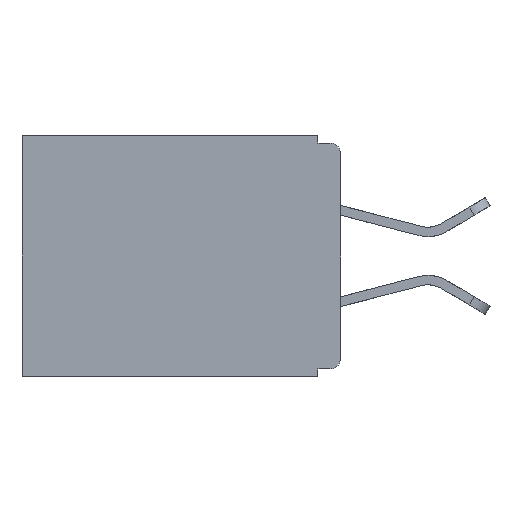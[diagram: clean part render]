
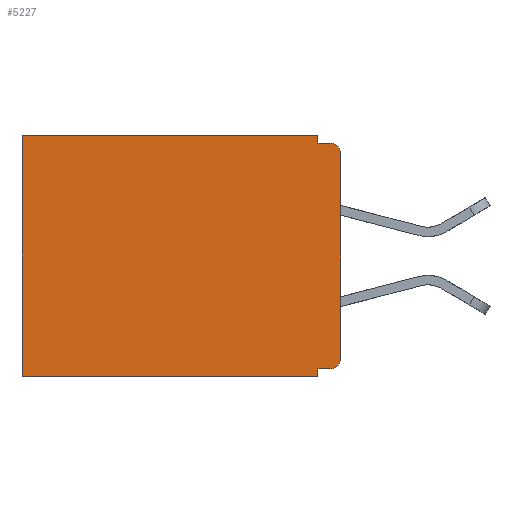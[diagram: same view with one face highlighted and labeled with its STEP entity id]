
A CAD part, left-side view. The second image highlights one B-rep face of the part: STEP entity #5227.
In plain terms, the highlighted planar face has unit normal (-1, 0, 0).
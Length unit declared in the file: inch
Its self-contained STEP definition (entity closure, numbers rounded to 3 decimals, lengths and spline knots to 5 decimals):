
#368 = VERTEX_POINT ( 'NONE', #8311 ) ;
#530 = VERTEX_POINT ( 'NONE', #10946 ) ;
#585 = AXIS2_PLACEMENT_3D ( 'NONE', #1080, #3379, #8536 ) ;
#915 = VERTEX_POINT ( 'NONE', #3968 ) ;
#994 = CARTESIAN_POINT ( 'NONE',  ( 0.3, 0., -0.33 ) ) ;
#1080 = CARTESIAN_POINT ( 'NONE',  ( 0.3, 0.015, -0.305 ) ) ;
#1088 = EDGE_CURVE ( 'NONE', #9975, #915, #9364, .T. ) ;
#1095 = ORIENTED_EDGE ( 'NONE', *, *, #3315, .F. ) ;
#1232 = LINE ( 'NONE', #8206, #9910 ) ;
#1527 = ORIENTED_EDGE ( 'NONE', *, *, #5737, .F. ) ;
#1800 = ORIENTED_EDGE ( 'NONE', *, *, #7945, .T. ) ;
#2013 = EDGE_CURVE ( 'NONE', #6006, #915, #11269, .T. ) ;
#2348 = CARTESIAN_POINT ( 'NONE',  ( 0.3, 0.437, -0.33 ) ) ;
#2437 = EDGE_LOOP ( 'NONE', ( #8509, #5768, #5359, #13763, #1800, #11108, #1527, #12391, #1095, #11787 ) ) ;
#2526 = LINE ( 'NONE', #6391, #11180 ) ;
#2609 = VECTOR ( 'NONE', #4242, 39.37008 ) ;
#2669 = CARTESIAN_POINT ( 'NONE',  ( 0.3, 0.031, -0.33 ) ) ;
#3148 = EDGE_CURVE ( 'NONE', #6006, #14381, #8460, .T. ) ;
#3163 = VECTOR ( 'NONE', #3804, 39.37008 ) ;
#3315 = EDGE_CURVE ( 'NONE', #9975, #7925, #3990, .T. ) ;
#3379 = DIRECTION ( 'NONE',  ( -1., 0., 0. ) ) ;
#3409 = VECTOR ( 'NONE', #7066, 39.37008 ) ;
#3683 = CARTESIAN_POINT ( 'NONE',  ( 0.3, 0., -0.32 ) ) ;
#3804 = DIRECTION ( 'NONE',  ( 0., 0., -1. ) ) ;
#3898 = DIRECTION ( 'NONE',  ( 0., 1., 0. ) ) ;
#3952 = CARTESIAN_POINT ( 'NONE',  ( 0.3, 0.031, -0.33 ) ) ;
#3968 = CARTESIAN_POINT ( 'NONE',  ( 0.3, 0., -0.305 ) ) ;
#3990 = LINE ( 'NONE', #3683, #6693 ) ;
#4228 = CARTESIAN_POINT ( 'NONE',  ( 0.3, 0., -0.33 ) ) ;
#4242 = DIRECTION ( 'NONE',  ( 0., 0., -1. ) ) ;
#4567 = VERTEX_POINT ( 'NONE', #3952 ) ;
#5057 = CARTESIAN_POINT ( 'NONE',  ( 0.3, 0.015, -0.01 ) ) ;
#5060 = CARTESIAN_POINT ( 'NONE',  ( 0.3, 0.031, -0.32 ) ) ;
#5227 = ADVANCED_FACE ( 'NONE', ( #8764 ), #5951, .F. ) ;
#5359 = ORIENTED_EDGE ( 'NONE', *, *, #6776, .F. ) ;
#5534 = EDGE_CURVE ( 'NONE', #6326, #8712, #2526, .T. ) ;
#5685 = CARTESIAN_POINT ( 'NONE',  ( 0.3, 0.437, 0. ) ) ;
#5737 = EDGE_CURVE ( 'NONE', #4567, #8712, #11700, .T. ) ;
#5768 = ORIENTED_EDGE ( 'NONE', *, *, #3148, .T. ) ;
#5951 = PLANE ( 'NONE',  #8265 ) ;
#6006 = VERTEX_POINT ( 'NONE', #10022 ) ;
#6097 = VECTOR ( 'NONE', #13013, 39.37008 ) ;
#6257 = LINE ( 'NONE', #2669, #3163 ) ;
#6326 = VERTEX_POINT ( 'NONE', #5685 ) ;
#6391 = CARTESIAN_POINT ( 'NONE',  ( 0.3, 0.437, -0.33 ) ) ;
#6445 = AXIS2_PLACEMENT_3D ( 'NONE', #10633, #7828, #7995 ) ;
#6693 = VECTOR ( 'NONE', #10478, 39.37008 ) ;
#6776 = EDGE_CURVE ( 'NONE', #530, #14381, #7347, .T. ) ;
#7066 = DIRECTION ( 'NONE',  ( 0., 1., 0. ) ) ;
#7347 = LINE ( 'NONE', #13477, #10270 ) ;
#7828 = DIRECTION ( 'NONE',  ( -1., 0., 0. ) ) ;
#7925 = VERTEX_POINT ( 'NONE', #5060 ) ;
#7945 = EDGE_CURVE ( 'NONE', #368, #6326, #1232, .T. ) ;
#7995 = DIRECTION ( 'NONE',  ( 0., 0., -1. ) ) ;
#8206 = CARTESIAN_POINT ( 'NONE',  ( 0.3, 0., 0. ) ) ;
#8265 = AXIS2_PLACEMENT_3D ( 'NONE', #12332, #8872, #9337 ) ;
#8311 = CARTESIAN_POINT ( 'NONE',  ( 0.3, 0.031, 0. ) ) ;
#8460 = CIRCLE ( 'NONE', #6445, 0.015 ) ;
#8509 = ORIENTED_EDGE ( 'NONE', *, *, #2013, .F. ) ;
#8536 = DIRECTION ( 'NONE',  ( 0., 0., -1. ) ) ;
#8610 = CARTESIAN_POINT ( 'NONE',  ( 0.3, 0.031, 0. ) ) ;
#8712 = VERTEX_POINT ( 'NONE', #2348 ) ;
#8764 = FACE_OUTER_BOUND ( 'NONE', #2437, .T. ) ;
#8823 = DIRECTION ( 'NONE',  ( 0., 0., -1. ) ) ;
#8872 = DIRECTION ( 'NONE',  ( 1., 0., 0. ) ) ;
#9337 = DIRECTION ( 'NONE',  ( 0., 0., -1. ) ) ;
#9364 = CIRCLE ( 'NONE', #585, 0.015 ) ;
#9394 = LINE ( 'NONE', #8610, #6097 ) ;
#9910 = VECTOR ( 'NONE', #3898, 39.37008 ) ;
#9975 = VERTEX_POINT ( 'NONE', #11405 ) ;
#10022 = CARTESIAN_POINT ( 'NONE',  ( 0.3, 0., -0.025 ) ) ;
#10270 = VECTOR ( 'NONE', #13642, 39.37008 ) ;
#10478 = DIRECTION ( 'NONE',  ( 0., 1., 0. ) ) ;
#10633 = CARTESIAN_POINT ( 'NONE',  ( 0.3, 0.015, -0.025 ) ) ;
#10946 = CARTESIAN_POINT ( 'NONE',  ( 0.3, 0.031, -0.01 ) ) ;
#11108 = ORIENTED_EDGE ( 'NONE', *, *, #5534, .T. ) ;
#11180 = VECTOR ( 'NONE', #8823, 39.37008 ) ;
#11269 = LINE ( 'NONE', #4228, #2609 ) ;
#11405 = CARTESIAN_POINT ( 'NONE',  ( 0.3, 0.015, -0.32 ) ) ;
#11700 = LINE ( 'NONE', #994, #3409 ) ;
#11787 = ORIENTED_EDGE ( 'NONE', *, *, #1088, .T. ) ;
#12332 = CARTESIAN_POINT ( 'NONE',  ( 0.3, 0., -0.33 ) ) ;
#12391 = ORIENTED_EDGE ( 'NONE', *, *, #14327, .F. ) ;
#13013 = DIRECTION ( 'NONE',  ( 0., 0., -1. ) ) ;
#13477 = CARTESIAN_POINT ( 'NONE',  ( 0.3, 0., -0.01 ) ) ;
#13642 = DIRECTION ( 'NONE',  ( 0., -1., 0. ) ) ;
#13736 = EDGE_CURVE ( 'NONE', #368, #530, #9394, .T. ) ;
#13763 = ORIENTED_EDGE ( 'NONE', *, *, #13736, .F. ) ;
#14327 = EDGE_CURVE ( 'NONE', #7925, #4567, #6257, .T. ) ;
#14381 = VERTEX_POINT ( 'NONE', #5057 ) ;
